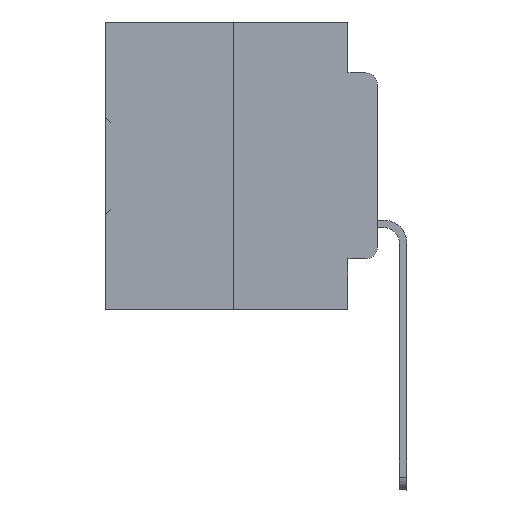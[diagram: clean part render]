
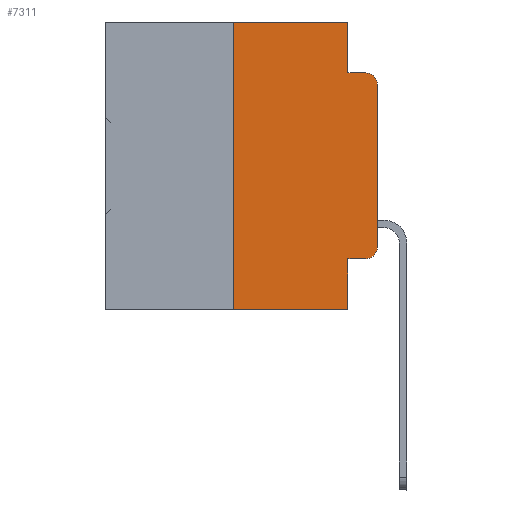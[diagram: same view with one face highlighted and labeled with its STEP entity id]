
A CAD part, left-side view. The second image highlights one B-rep face of the part: STEP entity #7311.
In plain terms, the highlighted planar face has unit normal (-1, 0, 0).
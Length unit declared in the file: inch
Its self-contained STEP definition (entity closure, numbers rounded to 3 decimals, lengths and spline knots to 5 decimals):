
#142 = VECTOR ( 'NONE', #11905, 39.37008 ) ;
#247 = DIRECTION ( 'NONE',  ( 0., 0., -1. ) ) ;
#1212 = VERTEX_POINT ( 'NONE', #23488 ) ;
#1465 = CARTESIAN_POINT ( 'NONE',  ( 0., 0.051, -0.4115 ) ) ;
#2748 = VECTOR ( 'NONE', #4882, 39.37008 ) ;
#2759 = DIRECTION ( 'NONE',  ( 0., 0., -1. ) ) ;
#4310 = LINE ( 'NONE', #15843, #8742 ) ;
#4507 = CARTESIAN_POINT ( 'NONE',  ( 0., 0.051, -0.4115 ) ) ;
#4521 = PLANE ( 'NONE',  #21984 ) ;
#4551 = ORIENTED_EDGE ( 'NONE', *, *, #12698, .T. ) ;
#4792 = CARTESIAN_POINT ( 'NONE',  ( 0., 0.02, -0.3915 ) ) ;
#4882 = DIRECTION ( 'NONE',  ( 0., -1., 0. ) ) ;
#5153 = VECTOR ( 'NONE', #36013, 39.37008 ) ;
#5157 = VERTEX_POINT ( 'NONE', #34731 ) ;
#5230 = EDGE_CURVE ( 'NONE', #7667, #1212, #26812, .T. ) ;
#5331 = CARTESIAN_POINT ( 'NONE',  ( 0., 0.051, -0.0885 ) ) ;
#6268 = CARTESIAN_POINT ( 'NONE',  ( 0., 0.051, 0. ) ) ;
#7311 = ADVANCED_FACE ( 'NONE', ( #13032 ), #4521, .F. ) ;
#7541 = EDGE_CURVE ( 'NONE', #19423, #25901, #14136, .T. ) ;
#7667 = VERTEX_POINT ( 'NONE', #32808 ) ;
#8086 = DIRECTION ( 'NONE',  ( 0., 0., 1. ) ) ;
#8102 = VECTOR ( 'NONE', #8086, 39.37008 ) ;
#8742 = VECTOR ( 'NONE', #12828, 39.37008 ) ;
#9060 = EDGE_CURVE ( 'NONE', #35824, #35899, #19032, .T. ) ;
#9395 = VERTEX_POINT ( 'NONE', #33707 ) ;
#9598 = ORIENTED_EDGE ( 'NONE', *, *, #16619, .F. ) ;
#10750 = DIRECTION ( 'NONE',  ( 0., 0., -1. ) ) ;
#10775 = CARTESIAN_POINT ( 'NONE',  ( 0., 0., -0.1085 ) ) ;
#11010 = LINE ( 'NONE', #5331, #34710 ) ;
#11905 = DIRECTION ( 'NONE',  ( 0., -1., 0. ) ) ;
#12068 = ORIENTED_EDGE ( 'NONE', *, *, #9060, .T. ) ;
#12698 = EDGE_CURVE ( 'NONE', #25901, #19561, #35444, .T. ) ;
#12828 = DIRECTION ( 'NONE',  ( 0., 0., 1. ) ) ;
#13032 = FACE_OUTER_BOUND ( 'NONE', #18546, .T. ) ;
#13189 = AXIS2_PLACEMENT_3D ( 'NONE', #25785, #22774, #2759 ) ;
#14136 = LINE ( 'NONE', #26204, #8102 ) ;
#14236 = VECTOR ( 'NONE', #28089, 39.37008 ) ;
#15293 = LINE ( 'NONE', #30015, #5153 ) ;
#15482 = CARTESIAN_POINT ( 'NONE',  ( 0., 0.02, -0.4115 ) ) ;
#15843 = CARTESIAN_POINT ( 'NONE',  ( 0., 0.25, 0. ) ) ;
#15927 = AXIS2_PLACEMENT_3D ( 'NONE', #4792, #36481, #21780 ) ;
#16619 = EDGE_CURVE ( 'NONE', #7667, #9395, #4310, .T. ) ;
#16693 = DIRECTION ( 'NONE',  ( 0., -1., 0. ) ) ;
#16805 = ORIENTED_EDGE ( 'NONE', *, *, #17674, .F. ) ;
#17674 = EDGE_CURVE ( 'NONE', #35991, #19561, #11010, .T. ) ;
#17771 = CARTESIAN_POINT ( 'NONE',  ( 0., 0.473, -0.5 ) ) ;
#18486 = VECTOR ( 'NONE', #247, 39.37008 ) ;
#18546 = EDGE_LOOP ( 'NONE', ( #18684, #4551, #16805, #28928, #28189, #9598, #32575, #27980, #12068, #30780 ) ) ;
#18684 = ORIENTED_EDGE ( 'NONE', *, *, #7541, .T. ) ;
#19032 = LINE ( 'NONE', #1465, #14236 ) ;
#19240 = LINE ( 'NONE', #30756, #2748 ) ;
#19423 = VERTEX_POINT ( 'NONE', #27808 ) ;
#19561 = VERTEX_POINT ( 'NONE', #34743 ) ;
#21780 = DIRECTION ( 'NONE',  ( 0., 0., -1. ) ) ;
#21984 = AXIS2_PLACEMENT_3D ( 'NONE', #22440, #30949, #10750 ) ;
#22440 = CARTESIAN_POINT ( 'NONE',  ( 0., 0.473, 0. ) ) ;
#22774 = DIRECTION ( 'NONE',  ( -1., 0., 0. ) ) ;
#23488 = CARTESIAN_POINT ( 'NONE',  ( 0., 0.051, -0.5 ) ) ;
#25785 = CARTESIAN_POINT ( 'NONE',  ( 0., 0.02, -0.1085 ) ) ;
#25901 = VERTEX_POINT ( 'NONE', #10775 ) ;
#26204 = CARTESIAN_POINT ( 'NONE',  ( 0., 0., 0. ) ) ;
#26812 = LINE ( 'NONE', #17771, #142 ) ;
#27808 = CARTESIAN_POINT ( 'NONE',  ( 0., 0., -0.3915 ) ) ;
#27980 = ORIENTED_EDGE ( 'NONE', *, *, #35835, .F. ) ;
#28089 = DIRECTION ( 'NONE',  ( 0., -1., 0. ) ) ;
#28189 = ORIENTED_EDGE ( 'NONE', *, *, #36015, .F. ) ;
#28928 = ORIENTED_EDGE ( 'NONE', *, *, #36593, .F. ) ;
#28992 = CARTESIAN_POINT ( 'NONE',  ( 0., 0.051, -0.0885 ) ) ;
#30015 = CARTESIAN_POINT ( 'NONE',  ( 0., 0.051, 0. ) ) ;
#30394 = CIRCLE ( 'NONE', #15927, 0.02 ) ;
#30756 = CARTESIAN_POINT ( 'NONE',  ( 0., 0.473, 0. ) ) ;
#30780 = ORIENTED_EDGE ( 'NONE', *, *, #34077, .T. ) ;
#30949 = DIRECTION ( 'NONE',  ( 1., 0., 0. ) ) ;
#32147 = LINE ( 'NONE', #6268, #18486 ) ;
#32575 = ORIENTED_EDGE ( 'NONE', *, *, #5230, .T. ) ;
#32808 = CARTESIAN_POINT ( 'NONE',  ( 0., 0.25, -0.5 ) ) ;
#33707 = CARTESIAN_POINT ( 'NONE',  ( 0., 0.25, 0. ) ) ;
#34077 = EDGE_CURVE ( 'NONE', #35899, #19423, #30394, .T. ) ;
#34710 = VECTOR ( 'NONE', #16693, 39.37008 ) ;
#34731 = CARTESIAN_POINT ( 'NONE',  ( 0., 0.051, 0. ) ) ;
#34743 = CARTESIAN_POINT ( 'NONE',  ( 0., 0.02, -0.0885 ) ) ;
#35444 = CIRCLE ( 'NONE', #13189, 0.02 ) ;
#35824 = VERTEX_POINT ( 'NONE', #4507 ) ;
#35835 = EDGE_CURVE ( 'NONE', #35824, #1212, #15293, .T. ) ;
#35899 = VERTEX_POINT ( 'NONE', #15482 ) ;
#35991 = VERTEX_POINT ( 'NONE', #28992 ) ;
#36013 = DIRECTION ( 'NONE',  ( 0., 0., -1. ) ) ;
#36015 = EDGE_CURVE ( 'NONE', #9395, #5157, #19240, .T. ) ;
#36481 = DIRECTION ( 'NONE',  ( -1., 0., 0. ) ) ;
#36593 = EDGE_CURVE ( 'NONE', #5157, #35991, #32147, .T. ) ;
